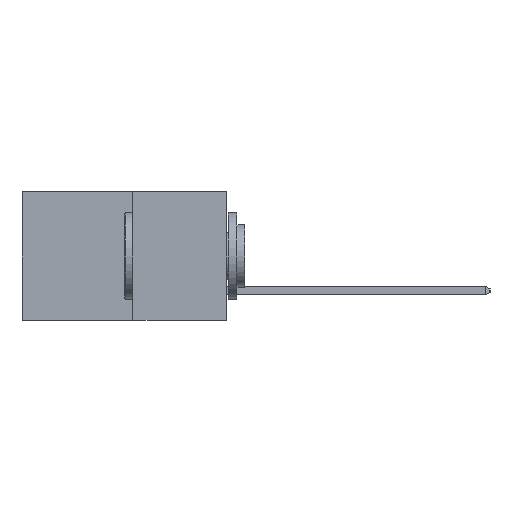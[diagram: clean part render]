
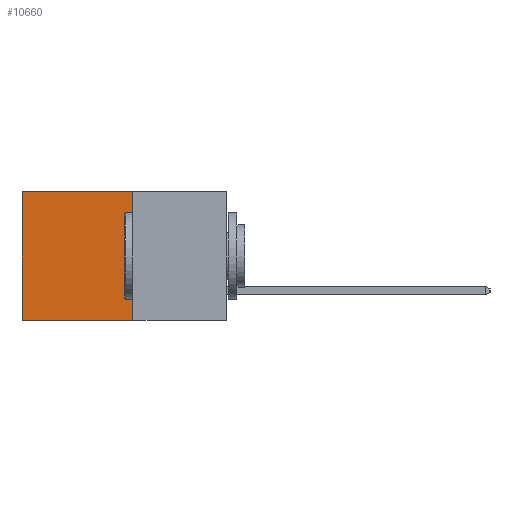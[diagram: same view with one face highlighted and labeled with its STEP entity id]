
A CAD part, left-side view. The second image highlights one B-rep face of the part: STEP entity #10660.
In plain terms, the highlighted planar face has unit normal (-1, 0, 0).
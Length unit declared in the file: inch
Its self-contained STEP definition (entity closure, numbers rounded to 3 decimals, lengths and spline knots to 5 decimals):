
#1379 = LINE ( 'NONE', #18123, #20822 ) ;
#1398 = AXIS2_PLACEMENT_3D ( 'NONE', #20372, #1599, #14869 ) ;
#1599 = DIRECTION ( 'NONE',  ( 1., 0., 0. ) ) ;
#5626 = VERTEX_POINT ( 'NONE', #19391 ) ;
#6884 = DIRECTION ( 'NONE',  ( 0., 1., 0. ) ) ;
#7423 = CARTESIAN_POINT ( 'NONE',  ( 0.277, 0.27, -0.37 ) ) ;
#7687 = VERTEX_POINT ( 'NONE', #21733 ) ;
#9287 = ORIENTED_EDGE ( 'NONE', *, *, #12100, .F. ) ;
#9690 = FACE_OUTER_BOUND ( 'NONE', #23654, .T. ) ;
#9815 = CARTESIAN_POINT ( 'NONE',  ( 0.277, 0.27, 0. ) ) ;
#9878 = ORIENTED_EDGE ( 'NONE', *, *, #10977, .T. ) ;
#10320 = DIRECTION ( 'NONE',  ( 0., 1., 0. ) ) ;
#10442 = ORIENTED_EDGE ( 'NONE', *, *, #17975, .F. ) ;
#10660 = ADVANCED_FACE ( 'NONE', ( #9690 ), #16627, .F. ) ;
#10893 = LINE ( 'NONE', #21473, #20209 ) ;
#10977 = EDGE_CURVE ( 'NONE', #5626, #7687, #22495, .T. ) ;
#11087 = EDGE_CURVE ( 'NONE', #13617, #5626, #10893, .T. ) ;
#11718 = VECTOR ( 'NONE', #13182, 39.37008 ) ;
#12100 = EDGE_CURVE ( 'NONE', #13617, #18559, #16658, .T. ) ;
#12670 = VECTOR ( 'NONE', #15558, 39.37008 ) ;
#13182 = DIRECTION ( 'NONE',  ( 0., 0., -1. ) ) ;
#13617 = VERTEX_POINT ( 'NONE', #9815 ) ;
#14869 = DIRECTION ( 'NONE',  ( 0., 0., -1. ) ) ;
#15558 = DIRECTION ( 'NONE',  ( 0., 0., -1. ) ) ;
#16627 = PLANE ( 'NONE',  #1398 ) ;
#16658 = LINE ( 'NONE', #7423, #11718 ) ;
#17416 = CARTESIAN_POINT ( 'NONE',  ( 0.277, 0.59, -0.37 ) ) ;
#17901 = ORIENTED_EDGE ( 'NONE', *, *, #11087, .T. ) ;
#17975 = EDGE_CURVE ( 'NONE', #18559, #7687, #1379, .T. ) ;
#18123 = CARTESIAN_POINT ( 'NONE',  ( 0.277, 0.27, -0.37 ) ) ;
#18176 = CARTESIAN_POINT ( 'NONE',  ( 0.277, 0.27, -0.37 ) ) ;
#18559 = VERTEX_POINT ( 'NONE', #18176 ) ;
#19391 = CARTESIAN_POINT ( 'NONE',  ( 0.277, 0.59, 0. ) ) ;
#20209 = VECTOR ( 'NONE', #10320, 39.37008 ) ;
#20372 = CARTESIAN_POINT ( 'NONE',  ( 0.277, 0.27, -0.37 ) ) ;
#20822 = VECTOR ( 'NONE', #6884, 39.37008 ) ;
#21473 = CARTESIAN_POINT ( 'NONE',  ( 0.277, 0.27, 0. ) ) ;
#21733 = CARTESIAN_POINT ( 'NONE',  ( 0.277, 0.59, -0.37 ) ) ;
#22495 = LINE ( 'NONE', #17416, #12670 ) ;
#23654 = EDGE_LOOP ( 'NONE', ( #9878, #10442, #9287, #17901 ) ) ;
